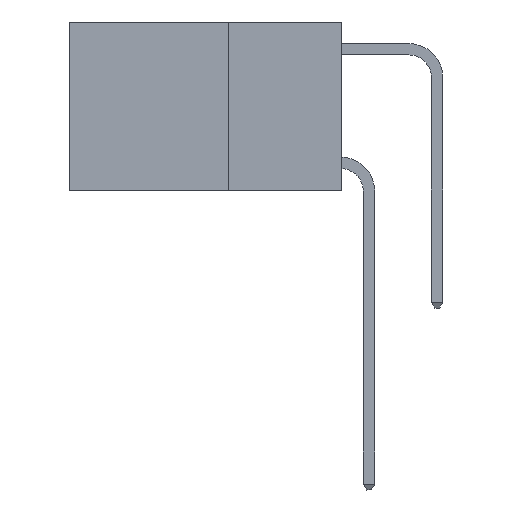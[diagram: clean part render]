
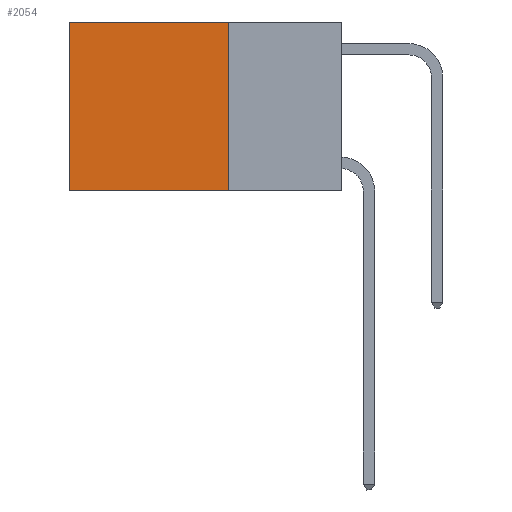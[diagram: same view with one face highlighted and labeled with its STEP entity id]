
A CAD part, left-side view. The second image highlights one B-rep face of the part: STEP entity #2054.
In plain terms, the highlighted planar face has unit normal (-1, 0, 0).
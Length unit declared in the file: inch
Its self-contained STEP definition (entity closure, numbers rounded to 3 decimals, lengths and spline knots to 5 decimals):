
#27 = ORIENTED_EDGE ( 'NONE', *, *, #2639, .T. ) ;
#936 = ORIENTED_EDGE ( 'NONE', *, *, #6187, .F. ) ;
#2054 = ADVANCED_FACE ( 'NONE', ( #11266 ), #8221, .F. ) ;
#2639 = EDGE_CURVE ( 'NONE', #3293, #2757, #2944, .T. ) ;
#2757 = VERTEX_POINT ( 'NONE', #4893 ) ;
#2889 = DIRECTION ( 'NONE',  ( 0., 1., 0. ) ) ;
#2891 = CARTESIAN_POINT ( 'NONE',  ( 0.2625, 0.25, 0. ) ) ;
#2944 = LINE ( 'NONE', #9009, #9563 ) ;
#3025 = ORIENTED_EDGE ( 'NONE', *, *, #10801, .F. ) ;
#3066 = CARTESIAN_POINT ( 'NONE',  ( 0.2625, 0.25, 0. ) ) ;
#3293 = VERTEX_POINT ( 'NONE', #5603 ) ;
#3940 = DIRECTION ( 'NONE',  ( 1., 0., 0. ) ) ;
#3954 = EDGE_LOOP ( 'NONE', ( #27, #936, #3025, #4057 ) ) ;
#4057 = ORIENTED_EDGE ( 'NONE', *, *, #5181, .T. ) ;
#4578 = VECTOR ( 'NONE', #5786, 39.37008 ) ;
#4746 = DIRECTION ( 'NONE',  ( 0., 0., -1. ) ) ;
#4893 = CARTESIAN_POINT ( 'NONE',  ( 0.2625, 0.6, -0.37 ) ) ;
#4931 = LINE ( 'NONE', #7668, #9256 ) ;
#5181 = EDGE_CURVE ( 'NONE', #7542, #3293, #11153, .T. ) ;
#5603 = CARTESIAN_POINT ( 'NONE',  ( 0.2625, 0.6, 0. ) ) ;
#5786 = DIRECTION ( 'NONE',  ( 0., 1., 0. ) ) ;
#5966 = DIRECTION ( 'NONE',  ( 0., 0., -1. ) ) ;
#6187 = EDGE_CURVE ( 'NONE', #9526, #2757, #7118, .T. ) ;
#7118 = LINE ( 'NONE', #11438, #11395 ) ;
#7445 = CARTESIAN_POINT ( 'NONE',  ( 0.2625, 0.25, -0.37 ) ) ;
#7542 = VERTEX_POINT ( 'NONE', #2891 ) ;
#7668 = CARTESIAN_POINT ( 'NONE',  ( 0.2625, 0.25, 0. ) ) ;
#8221 = PLANE ( 'NONE',  #11126 ) ;
#9009 = CARTESIAN_POINT ( 'NONE',  ( 0.2625, 0.6, 0. ) ) ;
#9256 = VECTOR ( 'NONE', #5966, 39.37008 ) ;
#9526 = VERTEX_POINT ( 'NONE', #7445 ) ;
#9563 = VECTOR ( 'NONE', #4746, 39.37008 ) ;
#9974 = DIRECTION ( 'NONE',  ( 0., 0., -1. ) ) ;
#10093 = CARTESIAN_POINT ( 'NONE',  ( 0.2625, 0.25, 0. ) ) ;
#10801 = EDGE_CURVE ( 'NONE', #7542, #9526, #4931, .T. ) ;
#11126 = AXIS2_PLACEMENT_3D ( 'NONE', #3066, #3940, #9974 ) ;
#11153 = LINE ( 'NONE', #10093, #4578 ) ;
#11266 = FACE_OUTER_BOUND ( 'NONE', #3954, .T. ) ;
#11395 = VECTOR ( 'NONE', #2889, 39.37008 ) ;
#11438 = CARTESIAN_POINT ( 'NONE',  ( 0.2625, 0.25, -0.37 ) ) ;
